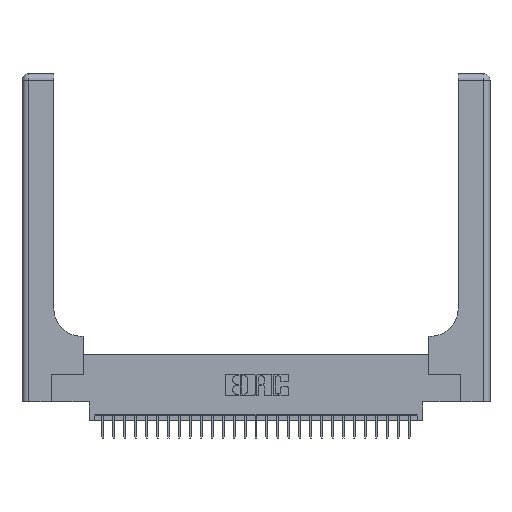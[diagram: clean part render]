
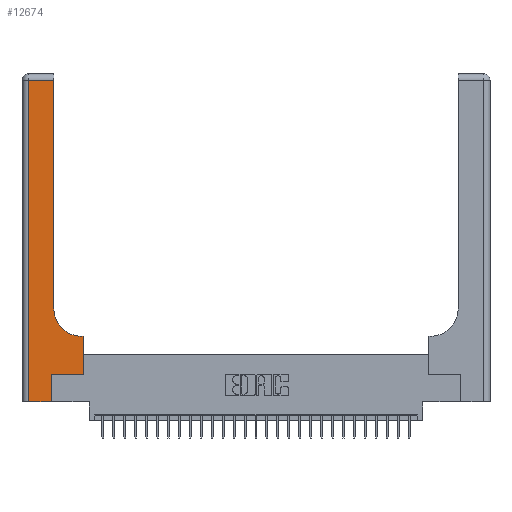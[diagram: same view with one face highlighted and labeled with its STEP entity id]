
A CAD part, top view. The second image highlights one B-rep face of the part: STEP entity #12674.
In plain terms, the highlighted planar face has unit normal (0, 0, 1).
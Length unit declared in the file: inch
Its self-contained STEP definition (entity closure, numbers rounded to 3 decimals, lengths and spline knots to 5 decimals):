
#80 = VERTEX_POINT ( 'NONE', #17556 ) ;
#1263 = ORIENTED_EDGE ( 'NONE', *, *, #21710, .T. ) ;
#1388 = CARTESIAN_POINT ( 'NONE',  ( 0.2915, 0.85, 0.37 ) ) ;
#1723 = DIRECTION ( 'NONE',  ( 1., 0., 0. ) ) ;
#1836 = AXIS2_PLACEMENT_3D ( 'NONE', #29335, #15608, #1723 ) ;
#2139 = ORIENTED_EDGE ( 'NONE', *, *, #19334, .T. ) ;
#2193 = LINE ( 'NONE', #12073, #7625 ) ;
#2984 = DIRECTION ( 'NONE',  ( -1., 0., 0. ) ) ;
#3092 = LINE ( 'NONE', #7757, #8560 ) ;
#3689 = EDGE_CURVE ( 'NONE', #13375, #29204, #19697, .T. ) ;
#3726 = VECTOR ( 'NONE', #29551, 39.37008 ) ;
#4150 = EDGE_CURVE ( 'NONE', #28184, #80, #9862, .T. ) ;
#4840 = ORIENTED_EDGE ( 'NONE', *, *, #16079, .T. ) ;
#5476 = FACE_OUTER_BOUND ( 'NONE', #14898, .T. ) ;
#5630 = VERTEX_POINT ( 'NONE', #1388 ) ;
#6148 = CARTESIAN_POINT ( 'NONE',  ( 0.269, 0., 0.37 ) ) ;
#6557 = VERTEX_POINT ( 'NONE', #26304 ) ;
#7625 = VECTOR ( 'NONE', #28170, 39.37008 ) ;
#7757 = CARTESIAN_POINT ( 'NONE',  ( 0.5585, 0.25, 0.37 ) ) ;
#7991 = DIRECTION ( 'NONE',  ( 1., 0., 0. ) ) ;
#7994 = VERTEX_POINT ( 'NONE', #17690 ) ;
#8560 = VECTOR ( 'NONE', #16967, 39.37008 ) ;
#9207 = ORIENTED_EDGE ( 'NONE', *, *, #4150, .T. ) ;
#9545 = CARTESIAN_POINT ( 'NONE',  ( 0.5585, 0.6, 0.37 ) ) ;
#9862 = LINE ( 'NONE', #16885, #16737 ) ;
#9947 = LINE ( 'NONE', #18051, #3726 ) ;
#10582 = DIRECTION ( 'NONE',  ( -1., 0., 0. ) ) ;
#10623 = LINE ( 'NONE', #24159, #16800 ) ;
#10786 = VECTOR ( 'NONE', #21590, 39.37008 ) ;
#11514 = LINE ( 'NONE', #16972, #10786 ) ;
#11555 = LINE ( 'NONE', #15155, #16999 ) ;
#12073 = CARTESIAN_POINT ( 'NONE',  ( 0.06, 3., 0.37 ) ) ;
#12169 = CARTESIAN_POINT ( 'NONE',  ( 0., 3., 0.37 ) ) ;
#12674 = ADVANCED_FACE ( 'NONE', ( #5476 ), #16748, .F. ) ;
#12832 = ORIENTED_EDGE ( 'NONE', *, *, #29627, .T. ) ;
#13375 = VERTEX_POINT ( 'NONE', #21713 ) ;
#14120 = EDGE_CURVE ( 'NONE', #24637, #23981, #11555, .T. ) ;
#14397 = ORIENTED_EDGE ( 'NONE', *, *, #17811, .T. ) ;
#14507 = DIRECTION ( 'NONE',  ( -1., 0., 0. ) ) ;
#14898 = EDGE_LOOP ( 'NONE', ( #1263, #9207, #14397, #2139, #29688, #19251, #4840, #21010, #12832 ) ) ;
#15155 = CARTESIAN_POINT ( 'NONE',  ( 0.2915, 0.6, 0.37 ) ) ;
#15608 = DIRECTION ( 'NONE',  ( 0., 0., -1. ) ) ;
#16079 = EDGE_CURVE ( 'NONE', #7994, #24637, #3092, .T. ) ;
#16737 = VECTOR ( 'NONE', #2984, 39.37008 ) ;
#16748 = PLANE ( 'NONE',  #24244 ) ;
#16800 = VECTOR ( 'NONE', #7991, 39.37008 ) ;
#16885 = CARTESIAN_POINT ( 'NONE',  ( 0., 2.94, 0.37 ) ) ;
#16967 = DIRECTION ( 'NONE',  ( 0., 1., 0. ) ) ;
#16972 = CARTESIAN_POINT ( 'NONE',  ( 0., 0., 0.37 ) ) ;
#16999 = VECTOR ( 'NONE', #10582, 39.37008 ) ;
#17556 = CARTESIAN_POINT ( 'NONE',  ( 0.06, 2.94, 0.37 ) ) ;
#17690 = CARTESIAN_POINT ( 'NONE',  ( 0.5585, 0.25, 0.37 ) ) ;
#17811 = EDGE_CURVE ( 'NONE', #80, #6557, #2193, .T. ) ;
#18051 = CARTESIAN_POINT ( 'NONE',  ( 0.2915, 3., 0.37 ) ) ;
#19239 = CIRCLE ( 'NONE', #1836, 0.25 ) ;
#19251 = ORIENTED_EDGE ( 'NONE', *, *, #22125, .T. ) ;
#19334 = EDGE_CURVE ( 'NONE', #6557, #13375, #11514, .T. ) ;
#19697 = LINE ( 'NONE', #6148, #23641 ) ;
#21010 = ORIENTED_EDGE ( 'NONE', *, *, #14120, .T. ) ;
#21590 = DIRECTION ( 'NONE',  ( 1., 0., 0. ) ) ;
#21710 = EDGE_CURVE ( 'NONE', #5630, #28184, #9947, .T. ) ;
#21713 = CARTESIAN_POINT ( 'NONE',  ( 0.269, 0., 0.37 ) ) ;
#22125 = EDGE_CURVE ( 'NONE', #29204, #7994, #10623, .T. ) ;
#23073 = CARTESIAN_POINT ( 'NONE',  ( 0.5415, 0.6, 0.37 ) ) ;
#23641 = VECTOR ( 'NONE', #26946, 39.37008 ) ;
#23981 = VERTEX_POINT ( 'NONE', #23073 ) ;
#24159 = CARTESIAN_POINT ( 'NONE',  ( 0.269, 0.25, 0.37 ) ) ;
#24244 = AXIS2_PLACEMENT_3D ( 'NONE', #12169, #28274, #14507 ) ;
#24487 = CARTESIAN_POINT ( 'NONE',  ( 0.2915, 2.94, 0.37 ) ) ;
#24637 = VERTEX_POINT ( 'NONE', #9545 ) ;
#25791 = CARTESIAN_POINT ( 'NONE',  ( 0.269, 0.25, 0.37 ) ) ;
#26304 = CARTESIAN_POINT ( 'NONE',  ( 0.06, 0., 0.37 ) ) ;
#26946 = DIRECTION ( 'NONE',  ( 0., 1., 0. ) ) ;
#28170 = DIRECTION ( 'NONE',  ( 0., -1., 0. ) ) ;
#28184 = VERTEX_POINT ( 'NONE', #24487 ) ;
#28274 = DIRECTION ( 'NONE',  ( 0., 0., -1. ) ) ;
#29204 = VERTEX_POINT ( 'NONE', #25791 ) ;
#29335 = CARTESIAN_POINT ( 'NONE',  ( 0.5415, 0.85, 0.37 ) ) ;
#29551 = DIRECTION ( 'NONE',  ( 0., 1., 0. ) ) ;
#29627 = EDGE_CURVE ( 'NONE', #23981, #5630, #19239, .T. ) ;
#29688 = ORIENTED_EDGE ( 'NONE', *, *, #3689, .T. ) ;
